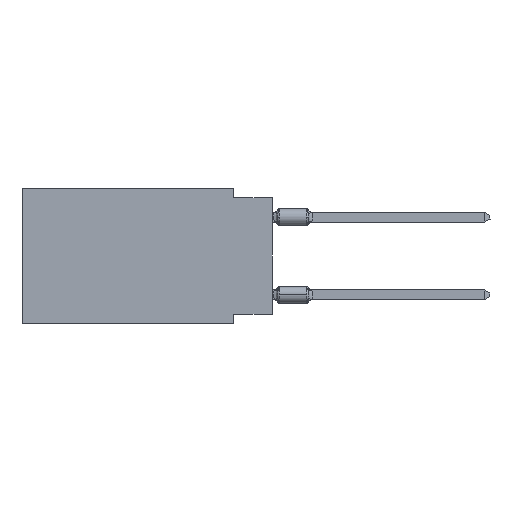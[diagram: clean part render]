
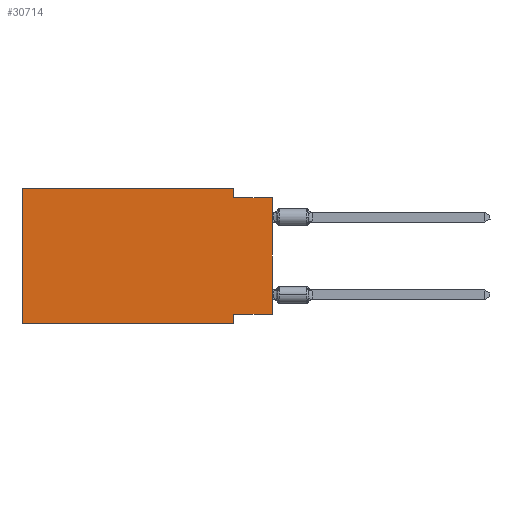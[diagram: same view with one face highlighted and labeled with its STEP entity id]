
A CAD part, left-side view. The second image highlights one B-rep face of the part: STEP entity #30714.
In plain terms, the highlighted planar face has unit normal (-1, 0, 0).
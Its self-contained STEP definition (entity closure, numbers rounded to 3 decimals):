
#2320 = LINE ( 'NONE', #17231, #8504 ) ;
#4445 = CARTESIAN_POINT ( 'NONE',  ( 0., 16.383, -8.89 ) ) ;
#4815 = DIRECTION ( 'NONE',  ( 0., -1., 0. ) ) ;
#4905 = LINE ( 'NONE', #43101, #39195 ) ;
#6643 = EDGE_CURVE ( 'NONE', #60405, #12685, #4905, .T. ) ;
#7428 = CARTESIAN_POINT ( 'NONE',  ( 0., 16.383, 0. ) ) ;
#8364 = CARTESIAN_POINT ( 'NONE',  ( 0., 16.383, 0. ) ) ;
#8504 = VECTOR ( 'NONE', #60429, 1000. ) ;
#8889 = DIRECTION ( 'NONE',  ( 1., 0., 0. ) ) ;
#8970 = CARTESIAN_POINT ( 'NONE',  ( 0., 0., -0.635 ) ) ;
#9209 = DIRECTION ( 'NONE',  ( 0., 0., -1. ) ) ;
#12685 = VERTEX_POINT ( 'NONE', #20930 ) ;
#13057 = LINE ( 'NONE', #50966, #13760 ) ;
#13760 = VECTOR ( 'NONE', #55933, 1000. ) ;
#14999 = LINE ( 'NONE', #4445, #38169 ) ;
#16466 = VERTEX_POINT ( 'NONE', #20985 ) ;
#17231 = CARTESIAN_POINT ( 'NONE',  ( 0., 0., 0. ) ) ;
#18507 = CARTESIAN_POINT ( 'NONE',  ( 0., 16.383, 0. ) ) ;
#19349 = ORIENTED_EDGE ( 'NONE', *, *, #59299, .F. ) ;
#20231 = VECTOR ( 'NONE', #4815, 1000. ) ;
#20930 = CARTESIAN_POINT ( 'NONE',  ( 0., 2.54, -0.635 ) ) ;
#20985 = CARTESIAN_POINT ( 'NONE',  ( 0., 2.54, -8.255 ) ) ;
#21492 = CARTESIAN_POINT ( 'NONE',  ( 0., 0., -0.635 ) ) ;
#21534 = ORIENTED_EDGE ( 'NONE', *, *, #41278, .T. ) ;
#23152 = LINE ( 'NONE', #18507, #20231 ) ;
#23267 = DIRECTION ( 'NONE',  ( 0., -1., 0. ) ) ;
#23803 = PLANE ( 'NONE',  #54438 ) ;
#23871 = DIRECTION ( 'NONE',  ( 0., 0., -1. ) ) ;
#24107 = DIRECTION ( 'NONE',  ( 0., 0., -1. ) ) ;
#25584 = EDGE_CURVE ( 'NONE', #35099, #60405, #23152, .T. ) ;
#27313 = VECTOR ( 'NONE', #23267, 1000. ) ;
#30714 = ADVANCED_FACE ( 'NONE', ( #38392 ), #23803, .F. ) ;
#33658 = DIRECTION ( 'NONE',  ( 0., -1., 0. ) ) ;
#34068 = LINE ( 'NONE', #8364, #38358 ) ;
#34841 = CARTESIAN_POINT ( 'NONE',  ( 0., 2.54, 0. ) ) ;
#35099 = VERTEX_POINT ( 'NONE', #7428 ) ;
#35622 = VERTEX_POINT ( 'NONE', #41212 ) ;
#37865 = LINE ( 'NONE', #8970, #27313 ) ;
#38000 = ORIENTED_EDGE ( 'NONE', *, *, #40617, .F. ) ;
#38112 = CARTESIAN_POINT ( 'NONE',  ( 0., 2.54, -8.89 ) ) ;
#38169 = VECTOR ( 'NONE', #33658, 1000. ) ;
#38358 = VECTOR ( 'NONE', #51256, 1000. ) ;
#38392 = FACE_OUTER_BOUND ( 'NONE', #39885, .T. ) ;
#39195 = VECTOR ( 'NONE', #23871, 1000. ) ;
#39885 = EDGE_LOOP ( 'NONE', ( #21534, #38000, #49127, #54505, #46024, #42489, #19349, #51653 ) ) ;
#40617 = EDGE_CURVE ( 'NONE', #12685, #51950, #37865, .T. ) ;
#41086 = CARTESIAN_POINT ( 'NONE',  ( 0., 16.383, -8.89 ) ) ;
#41212 = CARTESIAN_POINT ( 'NONE',  ( 0., 0., -8.255 ) ) ;
#41278 = EDGE_CURVE ( 'NONE', #35622, #51950, #2320, .T. ) ;
#42439 = EDGE_CURVE ( 'NONE', #50284, #35099, #34068, .T. ) ;
#42489 = ORIENTED_EDGE ( 'NONE', *, *, #54919, .T. ) ;
#42746 = LINE ( 'NONE', #38112, #54588 ) ;
#43101 = CARTESIAN_POINT ( 'NONE',  ( 0., 2.54, 0. ) ) ;
#46024 = ORIENTED_EDGE ( 'NONE', *, *, #42439, .F. ) ;
#48545 = VERTEX_POINT ( 'NONE', #50499 ) ;
#49127 = ORIENTED_EDGE ( 'NONE', *, *, #6643, .F. ) ;
#49551 = EDGE_CURVE ( 'NONE', #35622, #16466, #13057, .T. ) ;
#50284 = VERTEX_POINT ( 'NONE', #41086 ) ;
#50499 = CARTESIAN_POINT ( 'NONE',  ( 0., 2.54, -8.89 ) ) ;
#50966 = CARTESIAN_POINT ( 'NONE',  ( 0., 0., -8.255 ) ) ;
#51256 = DIRECTION ( 'NONE',  ( 0., 0., 1. ) ) ;
#51653 = ORIENTED_EDGE ( 'NONE', *, *, #49551, .F. ) ;
#51950 = VERTEX_POINT ( 'NONE', #21492 ) ;
#54438 = AXIS2_PLACEMENT_3D ( 'NONE', #57355, #8889, #24107 ) ;
#54505 = ORIENTED_EDGE ( 'NONE', *, *, #25584, .F. ) ;
#54588 = VECTOR ( 'NONE', #9209, 1000. ) ;
#54919 = EDGE_CURVE ( 'NONE', #50284, #48545, #14999, .T. ) ;
#55933 = DIRECTION ( 'NONE',  ( 0., 1., 0. ) ) ;
#57355 = CARTESIAN_POINT ( 'NONE',  ( 0., 16.383, 0. ) ) ;
#59299 = EDGE_CURVE ( 'NONE', #16466, #48545, #42746, .T. ) ;
#60405 = VERTEX_POINT ( 'NONE', #34841 ) ;
#60429 = DIRECTION ( 'NONE',  ( 0., 0., 1. ) ) ;
